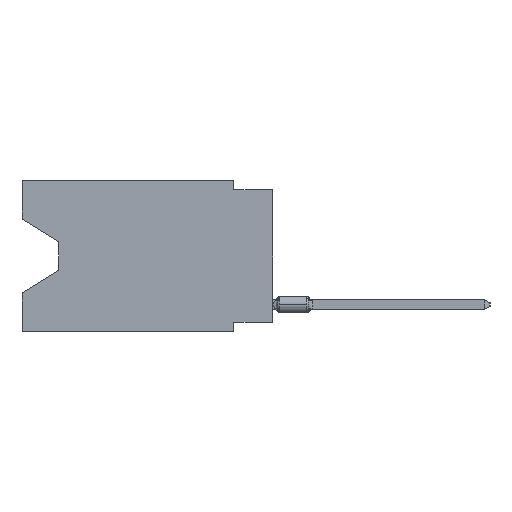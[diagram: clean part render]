
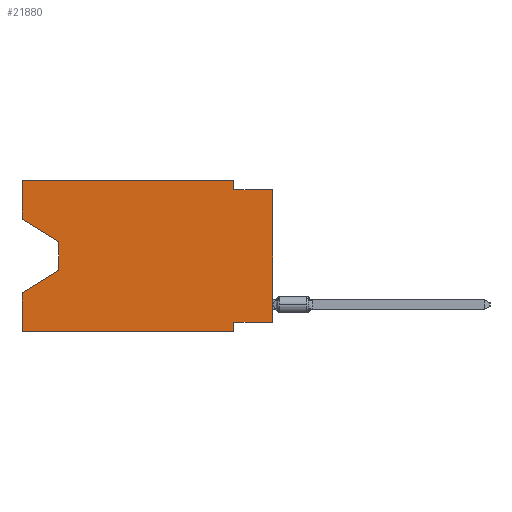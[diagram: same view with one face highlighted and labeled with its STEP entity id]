
A CAD part, left-side view. The second image highlights one B-rep face of the part: STEP entity #21880.
In plain terms, the highlighted planar face has unit normal (-1, 0, 0).
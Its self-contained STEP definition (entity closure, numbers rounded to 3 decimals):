
#753 = LINE ( 'NONE', #61404, #17341 ) ;
#760 = VECTOR ( 'NONE', #32311, 1000. ) ;
#998 = LINE ( 'NONE', #40391, #10914 ) ;
#1104 = VECTOR ( 'NONE', #37867, 1000. ) ;
#1473 = ORIENTED_EDGE ( 'NONE', *, *, #57003, .F. ) ;
#1750 = LINE ( 'NONE', #27306, #39648 ) ;
#1779 = LINE ( 'NONE', #31630, #1104 ) ;
#1858 = CARTESIAN_POINT ( 'NONE',  ( 0., 2.54, -0.635 ) ) ;
#2141 = LINE ( 'NONE', #56610, #760 ) ;
#2835 = LINE ( 'NONE', #43528, #56048 ) ;
#3751 = LINE ( 'NONE', #47745, #51068 ) ;
#3911 = CARTESIAN_POINT ( 'NONE',  ( 0., 2.54, -9.271 ) ) ;
#4098 = PLANE ( 'NONE',  #53791 ) ;
#4259 = EDGE_LOOP ( 'NONE', ( #28613, #16681, #39972, #15587, #15034, #14709, #1473, #14419, #24755, #13440, #60333, #57415 ) ) ;
#4427 = DIRECTION ( 'NONE',  ( 1., 0., 0. ) ) ;
#5054 = CARTESIAN_POINT ( 'NONE',  ( 0., 13.97, -5.893 ) ) ;
#5279 = DIRECTION ( 'NONE',  ( 0., 0., 1. ) ) ;
#5473 = LINE ( 'NONE', #10058, #15398 ) ;
#6920 = VERTEX_POINT ( 'NONE', #47078 ) ;
#7080 = VERTEX_POINT ( 'NONE', #28998 ) ;
#8361 = DIRECTION ( 'NONE',  ( 0., 0., -1. ) ) ;
#8384 = FACE_OUTER_BOUND ( 'NONE', #4259, .T. ) ;
#10058 = CARTESIAN_POINT ( 'NONE',  ( 0., 0., 0. ) ) ;
#10914 = VECTOR ( 'NONE', #5279, 1000. ) ;
#10962 = CARTESIAN_POINT ( 'NONE',  ( 0., 16.383, -9.906 ) ) ;
#11863 = CARTESIAN_POINT ( 'NONE',  ( 0., 16.383, 0. ) ) ;
#12139 = VERTEX_POINT ( 'NONE', #59809 ) ;
#13440 = ORIENTED_EDGE ( 'NONE', *, *, #28374, .F. ) ;
#13935 = DIRECTION ( 'NONE',  ( 0., 0., -1. ) ) ;
#13985 = VECTOR ( 'NONE', #22777, 1000. ) ;
#13987 = LINE ( 'NONE', #54355, #61781 ) ;
#14419 = ORIENTED_EDGE ( 'NONE', *, *, #53240, .T. ) ;
#14709 = ORIENTED_EDGE ( 'NONE', *, *, #52336, .F. ) ;
#15034 = ORIENTED_EDGE ( 'NONE', *, *, #52190, .T. ) ;
#15398 = VECTOR ( 'NONE', #60254, 1000. ) ;
#15587 = ORIENTED_EDGE ( 'NONE', *, *, #60487, .F. ) ;
#16184 = DIRECTION ( 'NONE',  ( 0., 0., 1. ) ) ;
#16681 = ORIENTED_EDGE ( 'NONE', *, *, #61663, .T. ) ;
#17018 = VECTOR ( 'NONE', #29524, 1000. ) ;
#17341 = VECTOR ( 'NONE', #36506, 1000. ) ;
#17488 = CARTESIAN_POINT ( 'NONE',  ( 0., 0., -9.271 ) ) ;
#18339 = VECTOR ( 'NONE', #55873, 1000. ) ;
#19009 = VERTEX_POINT ( 'NONE', #1858 ) ;
#20094 = VERTEX_POINT ( 'NONE', #63150 ) ;
#21880 = ADVANCED_FACE ( 'NONE', ( #8384 ), #4098, .F. ) ;
#22777 = DIRECTION ( 'NONE',  ( 0., -1., 0. ) ) ;
#23614 = CARTESIAN_POINT ( 'NONE',  ( 0., 0., -0.635 ) ) ;
#23932 = LINE ( 'NONE', #23614, #17018 ) ;
#24091 = CARTESIAN_POINT ( 'NONE',  ( 0., 16.383, 0. ) ) ;
#24755 = ORIENTED_EDGE ( 'NONE', *, *, #36799, .F. ) ;
#26332 = EDGE_CURVE ( 'NONE', #44027, #20094, #27057, .T. ) ;
#26744 = CARTESIAN_POINT ( 'NONE',  ( 0., 16.383, -2.546 ) ) ;
#27057 = LINE ( 'NONE', #47103, #13985 ) ;
#27306 = CARTESIAN_POINT ( 'NONE',  ( 0., 16.383, 0. ) ) ;
#27408 = VERTEX_POINT ( 'NONE', #5054 ) ;
#27600 = EDGE_CURVE ( 'NONE', #49573, #34434, #2835, .T. ) ;
#28374 = EDGE_CURVE ( 'NONE', #20094, #19009, #753, .T. ) ;
#28613 = ORIENTED_EDGE ( 'NONE', *, *, #27600, .T. ) ;
#28998 = CARTESIAN_POINT ( 'NONE',  ( 0., 2.54, -9.906 ) ) ;
#29524 = DIRECTION ( 'NONE',  ( 0., -1., 0. ) ) ;
#30060 = DIRECTION ( 'NONE',  ( 0., 0.855, -0.519 ) ) ;
#31630 = CARTESIAN_POINT ( 'NONE',  ( 0., 0., -9.271 ) ) ;
#32033 = DIRECTION ( 'NONE',  ( 0., -0.855, -0.519 ) ) ;
#32311 = DIRECTION ( 'NONE',  ( 0., -1., 0. ) ) ;
#34434 = VERTEX_POINT ( 'NONE', #44332 ) ;
#35552 = VERTEX_POINT ( 'NONE', #10962 ) ;
#35874 = LINE ( 'NONE', #45090, #18339 ) ;
#36506 = DIRECTION ( 'NONE',  ( 0., 0., -1. ) ) ;
#36799 = EDGE_CURVE ( 'NONE', #19009, #12139, #23932, .T. ) ;
#37867 = DIRECTION ( 'NONE',  ( 0., 1., 0. ) ) ;
#39149 = VERTEX_POINT ( 'NONE', #17488 ) ;
#39648 = VECTOR ( 'NONE', #16184, 1000. ) ;
#39972 = ORIENTED_EDGE ( 'NONE', *, *, #46256, .T. ) ;
#40391 = CARTESIAN_POINT ( 'NONE',  ( 0., 16.383, 0. ) ) ;
#43528 = CARTESIAN_POINT ( 'NONE',  ( 0., 16.383, -2.546 ) ) ;
#44027 = VERTEX_POINT ( 'NONE', #11863 ) ;
#44332 = CARTESIAN_POINT ( 'NONE',  ( 0., 13.97, -4.013 ) ) ;
#45090 = CARTESIAN_POINT ( 'NONE',  ( 0., 13.97, -4.013 ) ) ;
#46256 = EDGE_CURVE ( 'NONE', #27408, #6920, #13987, .T. ) ;
#47078 = CARTESIAN_POINT ( 'NONE',  ( 0., 16.383, -7.36 ) ) ;
#47103 = CARTESIAN_POINT ( 'NONE',  ( 0., 16.383, 0. ) ) ;
#47732 = VERTEX_POINT ( 'NONE', #3911 ) ;
#47745 = CARTESIAN_POINT ( 'NONE',  ( 0., 2.54, -9.906 ) ) ;
#49573 = VERTEX_POINT ( 'NONE', #26744 ) ;
#51068 = VECTOR ( 'NONE', #8361, 1000. ) ;
#52190 = EDGE_CURVE ( 'NONE', #35552, #7080, #2141, .T. ) ;
#52336 = EDGE_CURVE ( 'NONE', #47732, #7080, #3751, .T. ) ;
#53240 = EDGE_CURVE ( 'NONE', #39149, #12139, #5473, .T. ) ;
#53791 = AXIS2_PLACEMENT_3D ( 'NONE', #24091, #4427, #13935 ) ;
#53819 = EDGE_CURVE ( 'NONE', #49573, #44027, #1750, .T. ) ;
#54355 = CARTESIAN_POINT ( 'NONE',  ( 0., 13.97, -5.893 ) ) ;
#55873 = DIRECTION ( 'NONE',  ( 0., 0., -1. ) ) ;
#56048 = VECTOR ( 'NONE', #32033, 1000. ) ;
#56610 = CARTESIAN_POINT ( 'NONE',  ( 0., 16.383, -9.906 ) ) ;
#57003 = EDGE_CURVE ( 'NONE', #39149, #47732, #1779, .T. ) ;
#57415 = ORIENTED_EDGE ( 'NONE', *, *, #53819, .F. ) ;
#59809 = CARTESIAN_POINT ( 'NONE',  ( 0., 0., -0.635 ) ) ;
#60254 = DIRECTION ( 'NONE',  ( 0., 0., 1. ) ) ;
#60333 = ORIENTED_EDGE ( 'NONE', *, *, #26332, .F. ) ;
#60487 = EDGE_CURVE ( 'NONE', #35552, #6920, #998, .T. ) ;
#61404 = CARTESIAN_POINT ( 'NONE',  ( 0., 2.54, 0. ) ) ;
#61663 = EDGE_CURVE ( 'NONE', #34434, #27408, #35874, .T. ) ;
#61781 = VECTOR ( 'NONE', #30060, 1000. ) ;
#63150 = CARTESIAN_POINT ( 'NONE',  ( 0., 2.54, 0. ) ) ;
